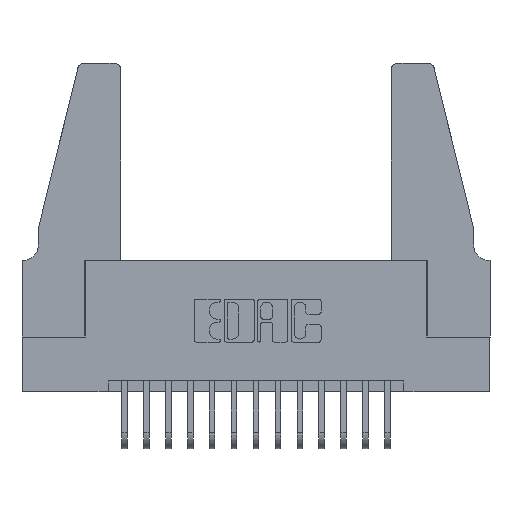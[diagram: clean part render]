
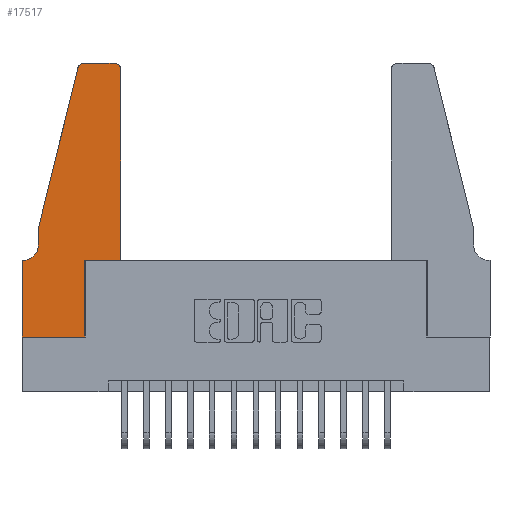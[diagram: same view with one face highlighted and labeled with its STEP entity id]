
A CAD part, top view. The second image highlights one B-rep face of the part: STEP entity #17517.
In plain terms, the highlighted planar face has unit normal (0, 0, 1).
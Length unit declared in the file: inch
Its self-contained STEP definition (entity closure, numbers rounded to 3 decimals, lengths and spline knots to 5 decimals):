
#331 = EDGE_CURVE ( 'NONE', #549, #8456, #17721, .T. ) ;
#513 = EDGE_CURVE ( 'NONE', #12191, #7647, #15736, .T. ) ;
#549 = VERTEX_POINT ( 'NONE', #5926 ) ;
#602 = CARTESIAN_POINT ( 'NONE',  ( 0.25487, 1.22718, 0.37 ) ) ;
#673 = CARTESIAN_POINT ( 'NONE',  ( 0.4205, 1.22, 0.37 ) ) ;
#862 = CARTESIAN_POINT ( 'NONE',  ( 0.2865, 0., 0.37 ) ) ;
#918 = VECTOR ( 'NONE', #2312, 39.37008 ) ;
#927 = CARTESIAN_POINT ( 'NONE',  ( 0., 0.35, 0.37 ) ) ;
#1183 = ORIENTED_EDGE ( 'NONE', *, *, #331, .T. ) ;
#1215 = LINE ( 'NONE', #3349, #11203 ) ;
#1253 = CARTESIAN_POINT ( 'NONE',  ( 0., 0., 0.37 ) ) ;
#1605 = VECTOR ( 'NONE', #8437, 39.37008 ) ;
#2312 = DIRECTION ( 'NONE',  ( 0., 1., 0. ) ) ;
#2612 = CARTESIAN_POINT ( 'NONE',  ( 0.284, 1.22, 0.37 ) ) ;
#2731 = ORIENTED_EDGE ( 'NONE', *, *, #11773, .T. ) ;
#2802 = CIRCLE ( 'NONE', #11506, 0.03 ) ;
#3349 = CARTESIAN_POINT ( 'NONE',  ( 0., 0., 0.37 ) ) ;
#3532 = VECTOR ( 'NONE', #13402, 39.37008 ) ;
#3617 = VERTEX_POINT ( 'NONE', #16543 ) ;
#3678 = DIRECTION ( 'NONE',  ( 1., 0., 0. ) ) ;
#3687 = EDGE_CURVE ( 'NONE', #15885, #15183, #6081, .T. ) ;
#3701 = CARTESIAN_POINT ( 'NONE',  ( 0.4505, 0.35, 0.37 ) ) ;
#3982 = DIRECTION ( 'NONE',  ( 0., 0., 1. ) ) ;
#4468 = EDGE_LOOP ( 'NONE', ( #1183, #2731, #17627, #9039, #13642, #17511, #16508, #11314, #13225, #8413, #4652, #5374 ) ) ;
#4652 = ORIENTED_EDGE ( 'NONE', *, *, #16786, .T. ) ;
#5351 = EDGE_CURVE ( 'NONE', #8025, #16048, #15794, .T. ) ;
#5374 = ORIENTED_EDGE ( 'NONE', *, *, #15375, .T. ) ;
#5766 = VECTOR ( 'NONE', #10860, 39.37008 ) ;
#5906 = LINE ( 'NONE', #16096, #13773 ) ;
#5926 = CARTESIAN_POINT ( 'NONE',  ( 0.4205, 1.25, 0.37 ) ) ;
#5964 = VERTEX_POINT ( 'NONE', #602 ) ;
#6081 = LINE ( 'NONE', #17543, #918 ) ;
#6189 = VERTEX_POINT ( 'NONE', #9866 ) ;
#6371 = DIRECTION ( 'NONE',  ( 0., 0., 1. ) ) ;
#6457 = CARTESIAN_POINT ( 'NONE',  ( 0.0755, 0.5, 0.37 ) ) ;
#6633 = VECTOR ( 'NONE', #6994, 39.37008 ) ;
#6994 = DIRECTION ( 'NONE',  ( -1., 0., 0. ) ) ;
#7272 = DIRECTION ( 'NONE',  ( 1., 0., 0. ) ) ;
#7647 = VERTEX_POINT ( 'NONE', #1253 ) ;
#7907 = CARTESIAN_POINT ( 'NONE',  ( 0.284, 1.25, 0.37 ) ) ;
#7997 = EDGE_CURVE ( 'NONE', #7647, #15885, #1215, .T. ) ;
#8025 = VERTEX_POINT ( 'NONE', #11488 ) ;
#8413 = ORIENTED_EDGE ( 'NONE', *, *, #14133, .T. ) ;
#8437 = DIRECTION ( 'NONE',  ( -1., 0., 0. ) ) ;
#8456 = VERTEX_POINT ( 'NONE', #7907 ) ;
#8696 = DIRECTION ( 'NONE',  ( 0., 0., 1. ) ) ;
#8970 = LINE ( 'NONE', #6457, #3532 ) ;
#9039 = ORIENTED_EDGE ( 'NONE', *, *, #12324, .T. ) ;
#9178 = CIRCLE ( 'NONE', #10140, 0.03 ) ;
#9651 = EDGE_CURVE ( 'NONE', #5964, #15559, #8970, .T. ) ;
#9866 = CARTESIAN_POINT ( 'NONE',  ( 0.4505, 0.35, 0.37 ) ) ;
#10105 = EDGE_CURVE ( 'NONE', #16048, #12191, #16215, .T. ) ;
#10140 = AXIS2_PLACEMENT_3D ( 'NONE', #673, #6371, #3678 ) ;
#10572 = VECTOR ( 'NONE', #14024, 39.37008 ) ;
#10739 = CARTESIAN_POINT ( 'NONE',  ( 0.0755, 0.5, 0.37 ) ) ;
#10781 = DIRECTION ( 'NONE',  ( 1., 0., 0. ) ) ;
#10860 = DIRECTION ( 'NONE',  ( 0., -1., 0. ) ) ;
#11178 = CARTESIAN_POINT ( 'NONE',  ( 0.2865, 0.35, 0.37 ) ) ;
#11203 = VECTOR ( 'NONE', #7272, 39.37008 ) ;
#11235 = CARTESIAN_POINT ( 'NONE',  ( 0.0755, 0.35, 0.37 ) ) ;
#11314 = ORIENTED_EDGE ( 'NONE', *, *, #7997, .T. ) ;
#11488 = CARTESIAN_POINT ( 'NONE',  ( 0.0755, 0.42, 0.37 ) ) ;
#11506 = AXIS2_PLACEMENT_3D ( 'NONE', #2612, #3982, #13886 ) ;
#11566 = CARTESIAN_POINT ( 'NONE',  ( 0., 0., 0.37 ) ) ;
#11603 = VECTOR ( 'NONE', #12080, 39.37008 ) ;
#11773 = EDGE_CURVE ( 'NONE', #8456, #5964, #2802, .T. ) ;
#12080 = DIRECTION ( 'NONE',  ( 0., 1., 0. ) ) ;
#12191 = VERTEX_POINT ( 'NONE', #927 ) ;
#12324 = EDGE_CURVE ( 'NONE', #15559, #8025, #16211, .T. ) ;
#12746 = CARTESIAN_POINT ( 'NONE',  ( 0.0055, 0.35, 0.37 ) ) ;
#12868 = DIRECTION ( 'NONE',  ( 0., 0., -1. ) ) ;
#13225 = ORIENTED_EDGE ( 'NONE', *, *, #3687, .T. ) ;
#13402 = DIRECTION ( 'NONE',  ( -0.239, -0.971, 0. ) ) ;
#13642 = ORIENTED_EDGE ( 'NONE', *, *, #5351, .T. ) ;
#13773 = VECTOR ( 'NONE', #10781, 39.37008 ) ;
#13886 = DIRECTION ( 'NONE',  ( 1., 0., 0. ) ) ;
#13932 = CARTESIAN_POINT ( 'NONE',  ( 0.0755, 0.5, 0.37 ) ) ;
#14024 = DIRECTION ( 'NONE',  ( 0., -1., 0. ) ) ;
#14133 = EDGE_CURVE ( 'NONE', #15183, #6189, #5906, .T. ) ;
#14290 = CARTESIAN_POINT ( 'NONE',  ( 0., 0.35, 0.37 ) ) ;
#14303 = AXIS2_PLACEMENT_3D ( 'NONE', #14290, #8696, #16937 ) ;
#14409 = DIRECTION ( 'NONE',  ( -1., 0., 0. ) ) ;
#14415 = AXIS2_PLACEMENT_3D ( 'NONE', #17228, #12868, #14409 ) ;
#15183 = VERTEX_POINT ( 'NONE', #11178 ) ;
#15351 = CARTESIAN_POINT ( 'NONE',  ( 0.2605, 1.25, 0.37 ) ) ;
#15375 = EDGE_CURVE ( 'NONE', #3617, #549, #9178, .T. ) ;
#15559 = VERTEX_POINT ( 'NONE', #10739 ) ;
#15639 = PLANE ( 'NONE',  #14303 ) ;
#15736 = LINE ( 'NONE', #11566, #10572 ) ;
#15794 = CIRCLE ( 'NONE', #14415, 0.07 ) ;
#15885 = VERTEX_POINT ( 'NONE', #862 ) ;
#16048 = VERTEX_POINT ( 'NONE', #12746 ) ;
#16096 = CARTESIAN_POINT ( 'NONE',  ( 0.4505, 0.35, 0.37 ) ) ;
#16119 = LINE ( 'NONE', #3701, #11603 ) ;
#16211 = LINE ( 'NONE', #13932, #5766 ) ;
#16215 = LINE ( 'NONE', #11235, #1605 ) ;
#16508 = ORIENTED_EDGE ( 'NONE', *, *, #513, .T. ) ;
#16543 = CARTESIAN_POINT ( 'NONE',  ( 0.4505, 1.22, 0.37 ) ) ;
#16786 = EDGE_CURVE ( 'NONE', #6189, #3617, #16119, .T. ) ;
#16937 = DIRECTION ( 'NONE',  ( 1., 0., 0. ) ) ;
#17019 = FACE_OUTER_BOUND ( 'NONE', #4468, .T. ) ;
#17228 = CARTESIAN_POINT ( 'NONE',  ( 0.0055, 0.42, 0.37 ) ) ;
#17511 = ORIENTED_EDGE ( 'NONE', *, *, #10105, .T. ) ;
#17517 = ADVANCED_FACE ( 'NONE', ( #17019 ), #15639, .T. ) ;
#17543 = CARTESIAN_POINT ( 'NONE',  ( 0.2865, 0.35, 0.37 ) ) ;
#17627 = ORIENTED_EDGE ( 'NONE', *, *, #9651, .T. ) ;
#17721 = LINE ( 'NONE', #15351, #6633 ) ;
